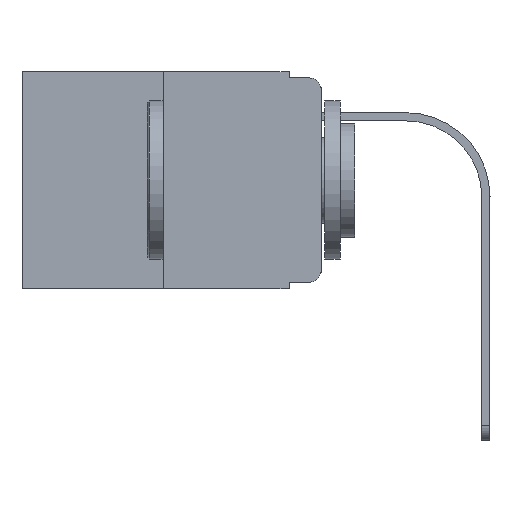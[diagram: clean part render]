
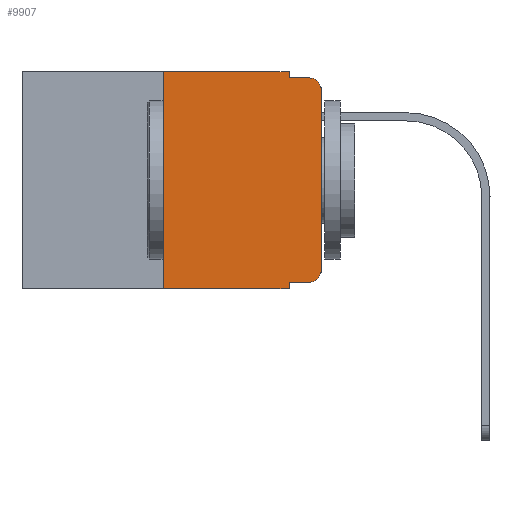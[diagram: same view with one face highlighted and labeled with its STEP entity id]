
A CAD part, left-side view. The second image highlights one B-rep face of the part: STEP entity #9907.
In plain terms, the highlighted planar face has unit normal (-1, 0, 0).
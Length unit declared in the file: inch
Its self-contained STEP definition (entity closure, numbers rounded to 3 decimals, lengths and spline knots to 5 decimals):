
#40 = EDGE_CURVE ( 'NONE', #18287, #9529, #12957, .T. ) ;
#79 = DIRECTION ( 'NONE',  ( 0., 0., -1. ) ) ;
#194 = LINE ( 'NONE', #8998, #17343 ) ;
#542 = EDGE_CURVE ( 'NONE', #6324, #19389, #15689, .T. ) ;
#809 = EDGE_CURVE ( 'NONE', #18287, #6324, #17060, .T. ) ;
#1077 = EDGE_CURVE ( 'NONE', #19389, #4427, #194, .T. ) ;
#1916 = CARTESIAN_POINT ( 'NONE',  ( 0., 0.02, -0.313 ) ) ;
#2051 = ORIENTED_EDGE ( 'NONE', *, *, #542, .T. ) ;
#2623 = EDGE_CURVE ( 'NONE', #14675, #15875, #17640, .T. ) ;
#2672 = CARTESIAN_POINT ( 'NONE',  ( 0., 0.051, 0. ) ) ;
#2999 = ORIENTED_EDGE ( 'NONE', *, *, #14434, .F. ) ;
#3360 = CARTESIAN_POINT ( 'NONE',  ( 0., 0.25, 0. ) ) ;
#3446 = ORIENTED_EDGE ( 'NONE', *, *, #15629, .F. ) ;
#3583 = CARTESIAN_POINT ( 'NONE',  ( 0., 0.02, -0.333 ) ) ;
#3680 = LINE ( 'NONE', #11318, #8049 ) ;
#4151 = CARTESIAN_POINT ( 'NONE',  ( 0., 0., -0.03 ) ) ;
#4211 = CARTESIAN_POINT ( 'NONE',  ( 0., 0.051, 0. ) ) ;
#4270 = ORIENTED_EDGE ( 'NONE', *, *, #14554, .T. ) ;
#4427 = VERTEX_POINT ( 'NONE', #4151 ) ;
#4733 = CARTESIAN_POINT ( 'NONE',  ( 0., 0.051, -0.343 ) ) ;
#4989 = DIRECTION ( 'NONE',  ( 0., 0., -1. ) ) ;
#5501 = VERTEX_POINT ( 'NONE', #18891 ) ;
#5865 = VECTOR ( 'NONE', #18339, 39.37008 ) ;
#6324 = VERTEX_POINT ( 'NONE', #3583 ) ;
#7072 = VECTOR ( 'NONE', #18597, 39.37008 ) ;
#7726 = CARTESIAN_POINT ( 'NONE',  ( 0., 0.051, -0.333 ) ) ;
#7873 = CARTESIAN_POINT ( 'NONE',  ( 0., 0.473, 0. ) ) ;
#8049 = VECTOR ( 'NONE', #17344, 39.37008 ) ;
#8682 = CARTESIAN_POINT ( 'NONE',  ( 0., 0., -0.313 ) ) ;
#8998 = CARTESIAN_POINT ( 'NONE',  ( 0., 0., 0. ) ) ;
#9529 = VERTEX_POINT ( 'NONE', #4733 ) ;
#9561 = AXIS2_PLACEMENT_3D ( 'NONE', #7873, #13849, #12164 ) ;
#9907 = ADVANCED_FACE ( 'NONE', ( #12468 ), #15432, .F. ) ;
#10199 = CARTESIAN_POINT ( 'NONE',  ( 0., 0.25, 0. ) ) ;
#10863 = CARTESIAN_POINT ( 'NONE',  ( 0., 0.051, 0. ) ) ;
#10909 = AXIS2_PLACEMENT_3D ( 'NONE', #15139, #13664, #79 ) ;
#11250 = ORIENTED_EDGE ( 'NONE', *, *, #14275, .T. ) ;
#11318 = CARTESIAN_POINT ( 'NONE',  ( 0., 0.473, -0.343 ) ) ;
#11614 = DIRECTION ( 'NONE',  ( 0., -1., 0. ) ) ;
#12164 = DIRECTION ( 'NONE',  ( 0., 0., -1. ) ) ;
#12468 = FACE_OUTER_BOUND ( 'NONE', #13228, .T. ) ;
#12957 = LINE ( 'NONE', #4211, #14184 ) ;
#13083 = LINE ( 'NONE', #14653, #18184 ) ;
#13228 = EDGE_LOOP ( 'NONE', ( #13902, #4270, #2999, #13586, #3446, #15341, #11250, #18270, #17472, #2051 ) ) ;
#13586 = ORIENTED_EDGE ( 'NONE', *, *, #16295, .F. ) ;
#13664 = DIRECTION ( 'NONE',  ( -1., 0., 0. ) ) ;
#13829 = DIRECTION ( 'NONE',  ( -1., 0., 0. ) ) ;
#13849 = DIRECTION ( 'NONE',  ( 1., 0., 0. ) ) ;
#13902 = ORIENTED_EDGE ( 'NONE', *, *, #1077, .T. ) ;
#13938 = LINE ( 'NONE', #10863, #7072 ) ;
#13962 = CARTESIAN_POINT ( 'NONE',  ( 0., 0.25, -0.343 ) ) ;
#14184 = VECTOR ( 'NONE', #16213, 39.37008 ) ;
#14275 = EDGE_CURVE ( 'NONE', #14675, #9529, #3680, .T. ) ;
#14390 = VERTEX_POINT ( 'NONE', #2672 ) ;
#14434 = EDGE_CURVE ( 'NONE', #16070, #5501, #13083, .T. ) ;
#14554 = EDGE_CURVE ( 'NONE', #4427, #5501, #19438, .T. ) ;
#14653 = CARTESIAN_POINT ( 'NONE',  ( 0., 0.051, -0.01 ) ) ;
#14675 = VERTEX_POINT ( 'NONE', #13962 ) ;
#15044 = AXIS2_PLACEMENT_3D ( 'NONE', #1916, #13829, #4989 ) ;
#15113 = CARTESIAN_POINT ( 'NONE',  ( 0., 0.051, -0.333 ) ) ;
#15139 = CARTESIAN_POINT ( 'NONE',  ( 0., 0.02, -0.03 ) ) ;
#15341 = ORIENTED_EDGE ( 'NONE', *, *, #2623, .F. ) ;
#15432 = PLANE ( 'NONE',  #9561 ) ;
#15629 = EDGE_CURVE ( 'NONE', #15875, #14390, #19118, .T. ) ;
#15689 = CIRCLE ( 'NONE', #15044, 0.02 ) ;
#15875 = VERTEX_POINT ( 'NONE', #3360 ) ;
#15959 = DIRECTION ( 'NONE',  ( 0., 0., 1. ) ) ;
#16070 = VERTEX_POINT ( 'NONE', #18918 ) ;
#16213 = DIRECTION ( 'NONE',  ( 0., 0., -1. ) ) ;
#16295 = EDGE_CURVE ( 'NONE', #14390, #16070, #13938, .T. ) ;
#16587 = VECTOR ( 'NONE', #15959, 39.37008 ) ;
#16647 = DIRECTION ( 'NONE',  ( 0., 0., 1. ) ) ;
#17060 = LINE ( 'NONE', #7726, #5865 ) ;
#17298 = VECTOR ( 'NONE', #11614, 39.37008 ) ;
#17343 = VECTOR ( 'NONE', #16647, 39.37008 ) ;
#17344 = DIRECTION ( 'NONE',  ( 0., -1., 0. ) ) ;
#17472 = ORIENTED_EDGE ( 'NONE', *, *, #809, .T. ) ;
#17636 = DIRECTION ( 'NONE',  ( 0., -1., 0. ) ) ;
#17640 = LINE ( 'NONE', #10199, #16587 ) ;
#18184 = VECTOR ( 'NONE', #17636, 39.37008 ) ;
#18270 = ORIENTED_EDGE ( 'NONE', *, *, #40, .F. ) ;
#18287 = VERTEX_POINT ( 'NONE', #15113 ) ;
#18339 = DIRECTION ( 'NONE',  ( 0., -1., 0. ) ) ;
#18597 = DIRECTION ( 'NONE',  ( 0., 0., -1. ) ) ;
#18891 = CARTESIAN_POINT ( 'NONE',  ( 0., 0.02, -0.01 ) ) ;
#18918 = CARTESIAN_POINT ( 'NONE',  ( 0., 0.051, -0.01 ) ) ;
#19118 = LINE ( 'NONE', #19300, #17298 ) ;
#19300 = CARTESIAN_POINT ( 'NONE',  ( 0., 0.473, 0. ) ) ;
#19389 = VERTEX_POINT ( 'NONE', #8682 ) ;
#19438 = CIRCLE ( 'NONE', #10909, 0.02 ) ;
